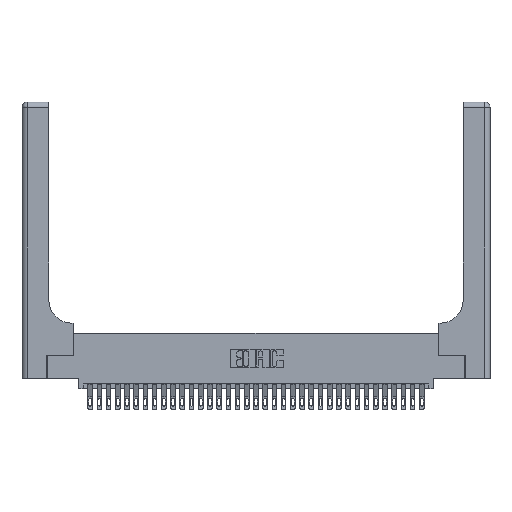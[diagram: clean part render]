
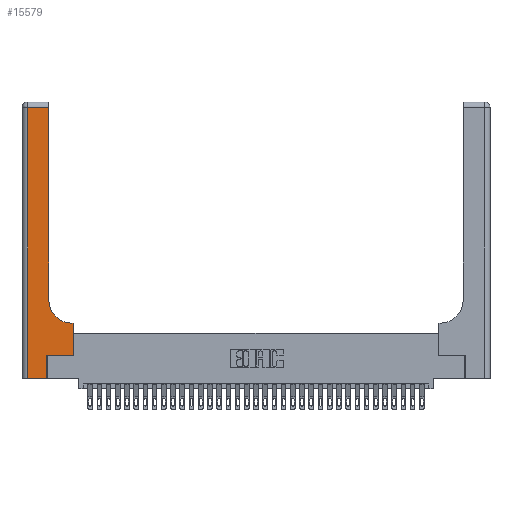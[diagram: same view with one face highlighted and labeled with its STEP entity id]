
A CAD part, top view. The second image highlights one B-rep face of the part: STEP entity #15579.
In plain terms, the highlighted planar face has unit normal (0, 0, 1).
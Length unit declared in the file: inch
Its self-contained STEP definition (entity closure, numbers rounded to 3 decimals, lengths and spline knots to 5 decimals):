
#5 = VERTEX_POINT ( 'NONE', #8488 ) ;
#642 = CARTESIAN_POINT ( 'NONE',  ( 0.5585, 0.6, 0.37 ) ) ;
#737 = CIRCLE ( 'NONE', #8924, 0.25 ) ;
#875 = VECTOR ( 'NONE', #23705, 39.37008 ) ;
#1107 = DIRECTION ( 'NONE',  ( 0., 0., -1. ) ) ;
#1143 = ORIENTED_EDGE ( 'NONE', *, *, #26969, .T. ) ;
#2173 = ORIENTED_EDGE ( 'NONE', *, *, #22848, .T. ) ;
#2432 = VECTOR ( 'NONE', #3181, 39.37008 ) ;
#2673 = FACE_OUTER_BOUND ( 'NONE', #31666, .T. ) ;
#2919 = CARTESIAN_POINT ( 'NONE',  ( 0.269, 0., 0.37 ) ) ;
#3181 = DIRECTION ( 'NONE',  ( 0., 1., 0. ) ) ;
#4026 = CARTESIAN_POINT ( 'NONE',  ( 0.5585, 0.25, 0.37 ) ) ;
#5479 = LINE ( 'NONE', #20114, #26523 ) ;
#6123 = CARTESIAN_POINT ( 'NONE',  ( 0.2915, 0.6, 0.37 ) ) ;
#6365 = DIRECTION ( 'NONE',  ( 1., 0., 0. ) ) ;
#6385 = VERTEX_POINT ( 'NONE', #14043 ) ;
#6715 = VERTEX_POINT ( 'NONE', #34427 ) ;
#6733 = EDGE_CURVE ( 'NONE', #5, #15536, #29204, .T. ) ;
#6789 = DIRECTION ( 'NONE',  ( 0., 1., 0. ) ) ;
#7646 = ORIENTED_EDGE ( 'NONE', *, *, #8533, .T. ) ;
#8349 = EDGE_CURVE ( 'NONE', #10641, #14337, #24383, .T. ) ;
#8488 = CARTESIAN_POINT ( 'NONE',  ( 0.269, 0.25, 0.37 ) ) ;
#8533 = EDGE_CURVE ( 'NONE', #15536, #9671, #32801, .T. ) ;
#8719 = DIRECTION ( 'NONE',  ( 0., 0., -1. ) ) ;
#8924 = AXIS2_PLACEMENT_3D ( 'NONE', #25143, #8719, #27863 ) ;
#9090 = CARTESIAN_POINT ( 'NONE',  ( 0.5585, 0.25, 0.37 ) ) ;
#9671 = VERTEX_POINT ( 'NONE', #642 ) ;
#10045 = CARTESIAN_POINT ( 'NONE',  ( 0.269, 0.25, 0.37 ) ) ;
#10436 = DIRECTION ( 'NONE',  ( 0., -1., 0. ) ) ;
#10606 = EDGE_CURVE ( 'NONE', #14337, #31847, #28042, .T. ) ;
#10641 = VERTEX_POINT ( 'NONE', #35307 ) ;
#10716 = CARTESIAN_POINT ( 'NONE',  ( 0., 2.94, 0.37 ) ) ;
#12550 = LINE ( 'NONE', #6123, #26216 ) ;
#12943 = CARTESIAN_POINT ( 'NONE',  ( 0.06, 2.94, 0.37 ) ) ;
#13520 = VECTOR ( 'NONE', #27101, 39.37008 ) ;
#14043 = CARTESIAN_POINT ( 'NONE',  ( 0.269, 0., 0.37 ) ) ;
#14337 = VERTEX_POINT ( 'NONE', #23112 ) ;
#15536 = VERTEX_POINT ( 'NONE', #9090 ) ;
#15579 = ADVANCED_FACE ( 'NONE', ( #2673 ), #31192, .F. ) ;
#17159 = EDGE_CURVE ( 'NONE', #6385, #5, #25781, .T. ) ;
#17353 = ORIENTED_EDGE ( 'NONE', *, *, #26024, .T. ) ;
#17600 = ORIENTED_EDGE ( 'NONE', *, *, #6733, .T. ) ;
#17632 = CARTESIAN_POINT ( 'NONE',  ( 0., 3., 0.37 ) ) ;
#17655 = ORIENTED_EDGE ( 'NONE', *, *, #17159, .T. ) ;
#18805 = ORIENTED_EDGE ( 'NONE', *, *, #10606, .T. ) ;
#19388 = VECTOR ( 'NONE', #22177, 39.37008 ) ;
#19446 = EDGE_CURVE ( 'NONE', #6715, #10641, #737, .T. ) ;
#19629 = ORIENTED_EDGE ( 'NONE', *, *, #19446, .T. ) ;
#19863 = DIRECTION ( 'NONE',  ( -1., 0., 0. ) ) ;
#20114 = CARTESIAN_POINT ( 'NONE',  ( 0., 0., 0.37 ) ) ;
#20383 = DIRECTION ( 'NONE',  ( -1., 0., 0. ) ) ;
#20779 = LINE ( 'NONE', #21382, #21624 ) ;
#21382 = CARTESIAN_POINT ( 'NONE',  ( 0.06, 3., 0.37 ) ) ;
#21624 = VECTOR ( 'NONE', #10436, 39.37008 ) ;
#22177 = DIRECTION ( 'NONE',  ( 0., 1., 0. ) ) ;
#22436 = CARTESIAN_POINT ( 'NONE',  ( 0.2915, 3., 0.37 ) ) ;
#22848 = EDGE_CURVE ( 'NONE', #32494, #6385, #5479, .T. ) ;
#23112 = CARTESIAN_POINT ( 'NONE',  ( 0.2915, 2.94, 0.37 ) ) ;
#23705 = DIRECTION ( 'NONE',  ( 1., 0., 0. ) ) ;
#24383 = LINE ( 'NONE', #22436, #2432 ) ;
#25143 = CARTESIAN_POINT ( 'NONE',  ( 0.5415, 0.85, 0.37 ) ) ;
#25657 = VECTOR ( 'NONE', #6789, 39.37008 ) ;
#25781 = LINE ( 'NONE', #2919, #19388 ) ;
#25904 = ORIENTED_EDGE ( 'NONE', *, *, #8349, .T. ) ;
#26024 = EDGE_CURVE ( 'NONE', #31847, #32494, #20779, .T. ) ;
#26216 = VECTOR ( 'NONE', #19863, 39.37008 ) ;
#26523 = VECTOR ( 'NONE', #6365, 39.37008 ) ;
#26969 = EDGE_CURVE ( 'NONE', #9671, #6715, #12550, .T. ) ;
#27101 = DIRECTION ( 'NONE',  ( -1., 0., 0. ) ) ;
#27863 = DIRECTION ( 'NONE',  ( 1., 0., 0. ) ) ;
#28042 = LINE ( 'NONE', #10716, #13520 ) ;
#29204 = LINE ( 'NONE', #10045, #875 ) ;
#29800 = AXIS2_PLACEMENT_3D ( 'NONE', #17632, #1107, #20383 ) ;
#31192 = PLANE ( 'NONE',  #29800 ) ;
#31378 = CARTESIAN_POINT ( 'NONE',  ( 0.06, 0., 0.37 ) ) ;
#31666 = EDGE_LOOP ( 'NONE', ( #25904, #18805, #17353, #2173, #17655, #17600, #7646, #1143, #19629 ) ) ;
#31847 = VERTEX_POINT ( 'NONE', #12943 ) ;
#32494 = VERTEX_POINT ( 'NONE', #31378 ) ;
#32801 = LINE ( 'NONE', #4026, #25657 ) ;
#34427 = CARTESIAN_POINT ( 'NONE',  ( 0.5415, 0.6, 0.37 ) ) ;
#35307 = CARTESIAN_POINT ( 'NONE',  ( 0.2915, 0.85, 0.37 ) ) ;
